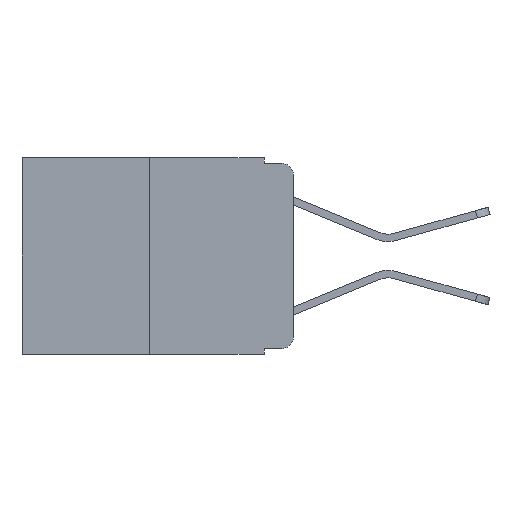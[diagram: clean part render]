
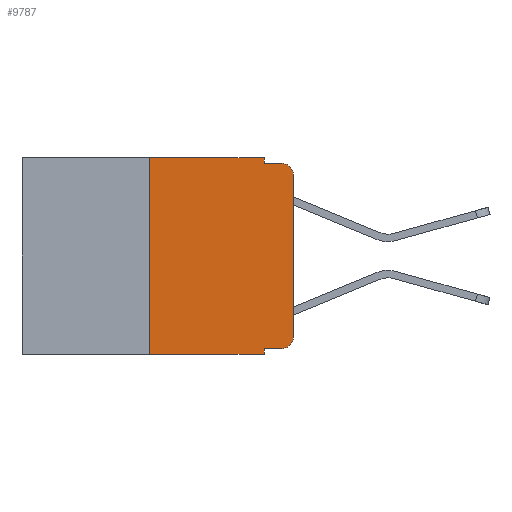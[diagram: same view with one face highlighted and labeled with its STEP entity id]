
A CAD part, left-side view. The second image highlights one B-rep face of the part: STEP entity #9787.
In plain terms, the highlighted planar face has unit normal (-1, 0, 0).
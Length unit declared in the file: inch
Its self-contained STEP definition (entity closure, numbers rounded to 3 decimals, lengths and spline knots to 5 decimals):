
#18 = CARTESIAN_POINT ( 'NONE',  ( 0., 0., 0. ) ) ;
#73 = VECTOR ( 'NONE', #5230, 39.37008 ) ;
#163 = AXIS2_PLACEMENT_3D ( 'NONE', #5612, #11624, #6504 ) ;
#314 = FACE_OUTER_BOUND ( 'NONE', #1328, .T. ) ;
#553 = DIRECTION ( 'NONE',  ( 0., 0., -1. ) ) ;
#591 = CARTESIAN_POINT ( 'NONE',  ( 0., 0.02, -0.313 ) ) ;
#639 = VERTEX_POINT ( 'NONE', #6798 ) ;
#662 = CARTESIAN_POINT ( 'NONE',  ( 0., 0.051, -0.01 ) ) ;
#692 = LINE ( 'NONE', #11105, #7810 ) ;
#699 = ORIENTED_EDGE ( 'NONE', *, *, #6432, .F. ) ;
#856 = CARTESIAN_POINT ( 'NONE',  ( 0., 0.25, -0.343 ) ) ;
#1186 = ORIENTED_EDGE ( 'NONE', *, *, #4882, .F. ) ;
#1243 = DIRECTION ( 'NONE',  ( 0., -1., 0. ) ) ;
#1268 = VECTOR ( 'NONE', #10586, 39.37008 ) ;
#1328 = EDGE_LOOP ( 'NONE', ( #1673, #8119, #1823, #1186, #699, #9979, #6497, #8912, #9317, #5171 ) ) ;
#1362 = CARTESIAN_POINT ( 'NONE',  ( 0., 0.051, -0.343 ) ) ;
#1384 = LINE ( 'NONE', #662, #10636 ) ;
#1498 = DIRECTION ( 'NONE',  ( 0., 0., -1. ) ) ;
#1569 = CIRCLE ( 'NONE', #8087, 0.02 ) ;
#1625 = DIRECTION ( 'NONE',  ( 0., 0., -1. ) ) ;
#1673 = ORIENTED_EDGE ( 'NONE', *, *, #2401, .T. ) ;
#1823 = ORIENTED_EDGE ( 'NONE', *, *, #3666, .F. ) ;
#2109 = EDGE_CURVE ( 'NONE', #3427, #4266, #3828, .T. ) ;
#2242 = VECTOR ( 'NONE', #2727, 39.37008 ) ;
#2256 = AXIS2_PLACEMENT_3D ( 'NONE', #591, #7128, #1625 ) ;
#2401 = EDGE_CURVE ( 'NONE', #9565, #6169, #6070, .T. ) ;
#2494 = CARTESIAN_POINT ( 'NONE',  ( 0., 0., -0.313 ) ) ;
#2727 = DIRECTION ( 'NONE',  ( 0., 0., -1. ) ) ;
#2794 = VERTEX_POINT ( 'NONE', #10147 ) ;
#3012 = LINE ( 'NONE', #10444, #73 ) ;
#3029 = EDGE_CURVE ( 'NONE', #6169, #9731, #1569, .T. ) ;
#3427 = VERTEX_POINT ( 'NONE', #11534 ) ;
#3474 = VECTOR ( 'NONE', #553, 39.37008 ) ;
#3664 = VERTEX_POINT ( 'NONE', #9772 ) ;
#3666 = EDGE_CURVE ( 'NONE', #3664, #9731, #1384, .T. ) ;
#3761 = VECTOR ( 'NONE', #3948, 39.37008 ) ;
#3828 = LINE ( 'NONE', #5134, #1268 ) ;
#3948 = DIRECTION ( 'NONE',  ( 0., -1., 0. ) ) ;
#4266 = VERTEX_POINT ( 'NONE', #8620 ) ;
#4584 = CARTESIAN_POINT ( 'NONE',  ( 0., 0.02, -0.01 ) ) ;
#4882 = EDGE_CURVE ( 'NONE', #639, #3664, #10508, .T. ) ;
#5002 = LINE ( 'NONE', #7266, #2242 ) ;
#5134 = CARTESIAN_POINT ( 'NONE',  ( 0., 0.051, -0.333 ) ) ;
#5171 = ORIENTED_EDGE ( 'NONE', *, *, #8936, .T. ) ;
#5230 = DIRECTION ( 'NONE',  ( 0., 0., 1. ) ) ;
#5398 = CIRCLE ( 'NONE', #2256, 0.02 ) ;
#5612 = CARTESIAN_POINT ( 'NONE',  ( 0., 0.473, 0. ) ) ;
#6059 = VERTEX_POINT ( 'NONE', #1362 ) ;
#6070 = LINE ( 'NONE', #18, #8984 ) ;
#6081 = EDGE_CURVE ( 'NONE', #6325, #2794, #3012, .T. ) ;
#6169 = VERTEX_POINT ( 'NONE', #10582 ) ;
#6325 = VERTEX_POINT ( 'NONE', #856 ) ;
#6432 = EDGE_CURVE ( 'NONE', #2794, #639, #10496, .T. ) ;
#6497 = ORIENTED_EDGE ( 'NONE', *, *, #7571, .T. ) ;
#6504 = DIRECTION ( 'NONE',  ( 0., 0., -1. ) ) ;
#6798 = CARTESIAN_POINT ( 'NONE',  ( 0., 0.051, 0. ) ) ;
#7092 = CARTESIAN_POINT ( 'NONE',  ( 0., 0.051, 0. ) ) ;
#7128 = DIRECTION ( 'NONE',  ( -1., 0., 0. ) ) ;
#7266 = CARTESIAN_POINT ( 'NONE',  ( 0., 0.051, 0. ) ) ;
#7571 = EDGE_CURVE ( 'NONE', #6325, #6059, #692, .T. ) ;
#7810 = VECTOR ( 'NONE', #1243, 39.37008 ) ;
#7888 = EDGE_CURVE ( 'NONE', #3427, #6059, #5002, .T. ) ;
#8087 = AXIS2_PLACEMENT_3D ( 'NONE', #11028, #11023, #1498 ) ;
#8119 = ORIENTED_EDGE ( 'NONE', *, *, #3029, .T. ) ;
#8620 = CARTESIAN_POINT ( 'NONE',  ( 0., 0.02, -0.333 ) ) ;
#8912 = ORIENTED_EDGE ( 'NONE', *, *, #7888, .F. ) ;
#8936 = EDGE_CURVE ( 'NONE', #4266, #9565, #5398, .T. ) ;
#8984 = VECTOR ( 'NONE', #11252, 39.37008 ) ;
#9280 = CARTESIAN_POINT ( 'NONE',  ( 0., 0.473, 0. ) ) ;
#9317 = ORIENTED_EDGE ( 'NONE', *, *, #2109, .T. ) ;
#9565 = VERTEX_POINT ( 'NONE', #2494 ) ;
#9731 = VERTEX_POINT ( 'NONE', #4584 ) ;
#9772 = CARTESIAN_POINT ( 'NONE',  ( 0., 0.051, -0.01 ) ) ;
#9787 = ADVANCED_FACE ( 'NONE', ( #314 ), #10799, .F. ) ;
#9979 = ORIENTED_EDGE ( 'NONE', *, *, #6081, .F. ) ;
#10147 = CARTESIAN_POINT ( 'NONE',  ( 0., 0.25, 0. ) ) ;
#10364 = DIRECTION ( 'NONE',  ( 0., -1., 0. ) ) ;
#10444 = CARTESIAN_POINT ( 'NONE',  ( 0., 0.25, 0. ) ) ;
#10496 = LINE ( 'NONE', #9280, #3761 ) ;
#10508 = LINE ( 'NONE', #7092, #3474 ) ;
#10582 = CARTESIAN_POINT ( 'NONE',  ( 0., 0., -0.03 ) ) ;
#10586 = DIRECTION ( 'NONE',  ( 0., -1., 0. ) ) ;
#10636 = VECTOR ( 'NONE', #10364, 39.37008 ) ;
#10799 = PLANE ( 'NONE',  #163 ) ;
#11023 = DIRECTION ( 'NONE',  ( -1., 0., 0. ) ) ;
#11028 = CARTESIAN_POINT ( 'NONE',  ( 0., 0.02, -0.03 ) ) ;
#11105 = CARTESIAN_POINT ( 'NONE',  ( 0., 0.473, -0.343 ) ) ;
#11252 = DIRECTION ( 'NONE',  ( 0., 0., 1. ) ) ;
#11534 = CARTESIAN_POINT ( 'NONE',  ( 0., 0.051, -0.333 ) ) ;
#11624 = DIRECTION ( 'NONE',  ( 1., 0., 0. ) ) ;
